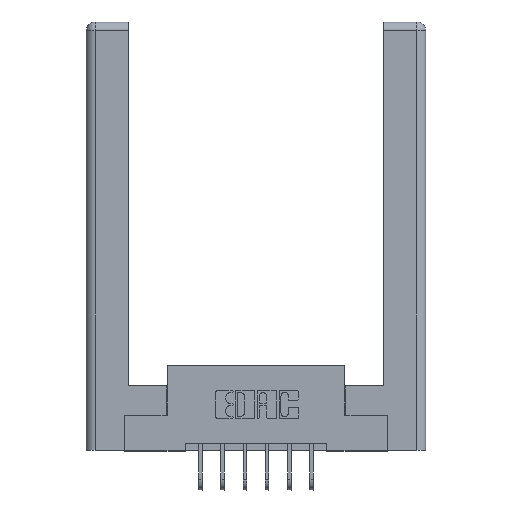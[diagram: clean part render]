
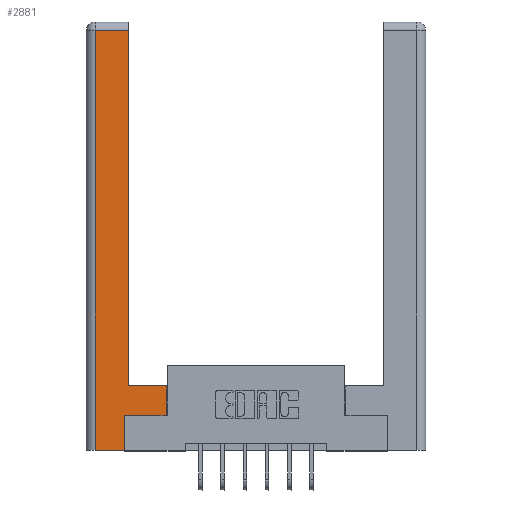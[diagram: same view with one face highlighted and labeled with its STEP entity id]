
A CAD part, top view. The second image highlights one B-rep face of the part: STEP entity #2881.
In plain terms, the highlighted planar face has unit normal (0, 0, 1).
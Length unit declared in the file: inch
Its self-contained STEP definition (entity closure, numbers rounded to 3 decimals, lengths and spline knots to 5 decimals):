
#136 = CARTESIAN_POINT ( 'NONE',  ( 0., 0., 0. ) ) ;
#941 = CARTESIAN_POINT ( 'NONE',  ( 0.265, 0.245, 0. ) ) ;
#976 = DIRECTION ( 'NONE',  ( 1., 0., 0. ) ) ;
#995 = CARTESIAN_POINT ( 'NONE',  ( 0.0615, 0., 0. ) ) ;
#1175 = DIRECTION ( 'NONE',  ( 0., -1., 0. ) ) ;
#1305 = VERTEX_POINT ( 'NONE', #995 ) ;
#1561 = VERTEX_POINT ( 'NONE', #941 ) ;
#1802 = DIRECTION ( 'NONE',  ( 0., 0., -1. ) ) ;
#1818 = VECTOR ( 'NONE', #11036, 39.37008 ) ;
#1849 = CARTESIAN_POINT ( 'NONE',  ( 0.565, 0.245, 0. ) ) ;
#2055 = VECTOR ( 'NONE', #976, 39.37008 ) ;
#2182 = CARTESIAN_POINT ( 'NONE',  ( 0.265, 0.245, 0. ) ) ;
#2241 = AXIS2_PLACEMENT_3D ( 'NONE', #136, #1802, #9219 ) ;
#2393 = LINE ( 'NONE', #2473, #9609 ) ;
#2473 = CARTESIAN_POINT ( 'NONE',  ( 0.295, 3., 0. ) ) ;
#2545 = EDGE_CURVE ( 'NONE', #9178, #9262, #4259, .T. ) ;
#2584 = VECTOR ( 'NONE', #3880, 39.37008 ) ;
#2881 = ADVANCED_FACE ( 'NONE', ( #11279 ), #7294, .F. ) ;
#3240 = CARTESIAN_POINT ( 'NONE',  ( 0.565, 0.45, 0. ) ) ;
#3268 = VERTEX_POINT ( 'NONE', #4395 ) ;
#3420 = EDGE_LOOP ( 'NONE', ( #10774, #4571, #9412, #6171, #11339, #5812, #8006, #4497 ) ) ;
#3880 = DIRECTION ( 'NONE',  ( 1., 0., 0. ) ) ;
#3914 = EDGE_CURVE ( 'NONE', #9262, #1305, #8269, .T. ) ;
#3951 = CARTESIAN_POINT ( 'NONE',  ( 0.0615, 2.94, 0. ) ) ;
#4076 = LINE ( 'NONE', #2182, #5630 ) ;
#4158 = DIRECTION ( 'NONE',  ( -1., 0., 0. ) ) ;
#4259 = LINE ( 'NONE', #10943, #1818 ) ;
#4395 = CARTESIAN_POINT ( 'NONE',  ( 0.565, 0.45, 0. ) ) ;
#4477 = LINE ( 'NONE', #1849, #2055 ) ;
#4497 = ORIENTED_EDGE ( 'NONE', *, *, #6446, .T. ) ;
#4571 = ORIENTED_EDGE ( 'NONE', *, *, #2545, .T. ) ;
#4618 = EDGE_CURVE ( 'NONE', #6960, #1561, #4076, .T. ) ;
#5078 = DIRECTION ( 'NONE',  ( 0., 1., 0. ) ) ;
#5201 = LINE ( 'NONE', #3240, #10827 ) ;
#5602 = VERTEX_POINT ( 'NONE', #9464 ) ;
#5630 = VECTOR ( 'NONE', #5766, 39.37008 ) ;
#5766 = DIRECTION ( 'NONE',  ( 0., 1., 0. ) ) ;
#5812 = ORIENTED_EDGE ( 'NONE', *, *, #9782, .T. ) ;
#6171 = ORIENTED_EDGE ( 'NONE', *, *, #11200, .T. ) ;
#6402 = LINE ( 'NONE', #6840, #10607 ) ;
#6446 = EDGE_CURVE ( 'NONE', #3268, #5602, #6402, .T. ) ;
#6607 = CARTESIAN_POINT ( 'NONE',  ( 0.0615, 0., 0. ) ) ;
#6755 = CARTESIAN_POINT ( 'NONE',  ( 0.265, 0., 0. ) ) ;
#6813 = EDGE_CURVE ( 'NONE', #5602, #9178, #2393, .T. ) ;
#6840 = CARTESIAN_POINT ( 'NONE',  ( 0.295, 0.45, 0. ) ) ;
#6960 = VERTEX_POINT ( 'NONE', #7309 ) ;
#7294 = PLANE ( 'NONE',  #2241 ) ;
#7309 = CARTESIAN_POINT ( 'NONE',  ( 0.265, 0., 0. ) ) ;
#8006 = ORIENTED_EDGE ( 'NONE', *, *, #9482, .T. ) ;
#8220 = LINE ( 'NONE', #6755, #2584 ) ;
#8269 = LINE ( 'NONE', #6607, #9564 ) ;
#8925 = CARTESIAN_POINT ( 'NONE',  ( 0.295, 2.94, 0. ) ) ;
#9178 = VERTEX_POINT ( 'NONE', #8925 ) ;
#9219 = DIRECTION ( 'NONE',  ( -1., 0., 0. ) ) ;
#9262 = VERTEX_POINT ( 'NONE', #3951 ) ;
#9412 = ORIENTED_EDGE ( 'NONE', *, *, #3914, .T. ) ;
#9464 = CARTESIAN_POINT ( 'NONE',  ( 0.295, 0.45, 0. ) ) ;
#9482 = EDGE_CURVE ( 'NONE', #10487, #3268, #5201, .T. ) ;
#9564 = VECTOR ( 'NONE', #1175, 39.37008 ) ;
#9609 = VECTOR ( 'NONE', #5078, 39.37008 ) ;
#9782 = EDGE_CURVE ( 'NONE', #1561, #10487, #4477, .T. ) ;
#10487 = VERTEX_POINT ( 'NONE', #10629 ) ;
#10607 = VECTOR ( 'NONE', #4158, 39.37008 ) ;
#10629 = CARTESIAN_POINT ( 'NONE',  ( 0.565, 0.245, 0. ) ) ;
#10774 = ORIENTED_EDGE ( 'NONE', *, *, #6813, .T. ) ;
#10827 = VECTOR ( 'NONE', #11487, 39.37008 ) ;
#10943 = CARTESIAN_POINT ( 'NONE',  ( 0.0615, 2.94, 0. ) ) ;
#11036 = DIRECTION ( 'NONE',  ( -1., 0., 0. ) ) ;
#11200 = EDGE_CURVE ( 'NONE', #1305, #6960, #8220, .T. ) ;
#11279 = FACE_OUTER_BOUND ( 'NONE', #3420, .T. ) ;
#11339 = ORIENTED_EDGE ( 'NONE', *, *, #4618, .T. ) ;
#11487 = DIRECTION ( 'NONE',  ( 0., 1., 0. ) ) ;
